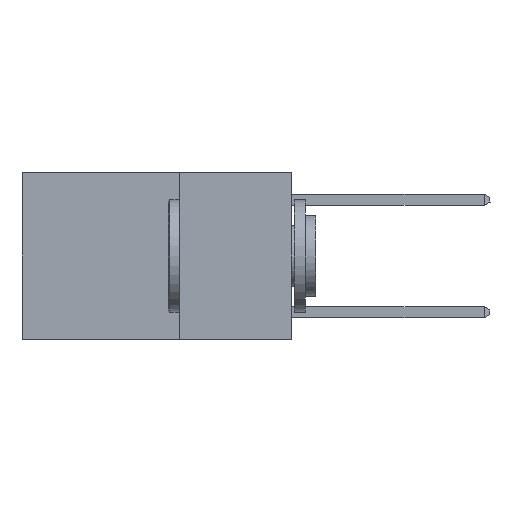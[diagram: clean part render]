
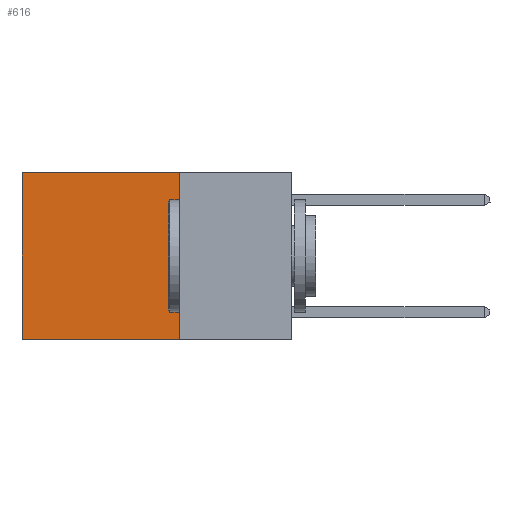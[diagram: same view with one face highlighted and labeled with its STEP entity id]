
A CAD part, left-side view. The second image highlights one B-rep face of the part: STEP entity #616.
In plain terms, the highlighted planar face has unit normal (-1, 0, 0).
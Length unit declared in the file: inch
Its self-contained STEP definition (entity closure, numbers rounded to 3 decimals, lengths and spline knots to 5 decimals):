
#616 = ADVANCED_FACE ( 'NONE', ( #10495 ), #8741, .F. ) ;
#1155 = DIRECTION ( 'NONE',  ( 1., 0., 0. ) ) ;
#2367 = DIRECTION ( 'NONE',  ( 0., 0., -1. ) ) ;
#2656 = LINE ( 'NONE', #16174, #15513 ) ;
#3738 = CARTESIAN_POINT ( 'NONE',  ( 0.2625, 0.6, 0. ) ) ;
#3993 = EDGE_CURVE ( 'NONE', #8483, #4294, #12483, .T. ) ;
#4294 = VERTEX_POINT ( 'NONE', #6613 ) ;
#4407 = AXIS2_PLACEMENT_3D ( 'NONE', #13640, #1155, #17614 ) ;
#5126 = CARTESIAN_POINT ( 'NONE',  ( 0.2625, 0.6, 0. ) ) ;
#6286 = ORIENTED_EDGE ( 'NONE', *, *, #8292, .T. ) ;
#6333 = DIRECTION ( 'NONE',  ( 0., 0., -1. ) ) ;
#6613 = CARTESIAN_POINT ( 'NONE',  ( 0.2625, 0.25, -0.37 ) ) ;
#6821 = EDGE_LOOP ( 'NONE', ( #9517, #14173, #14596, #6286 ) ) ;
#7365 = VECTOR ( 'NONE', #2367, 39.37008 ) ;
#7844 = VECTOR ( 'NONE', #6333, 39.37008 ) ;
#8292 = EDGE_CURVE ( 'NONE', #8483, #14912, #2656, .T. ) ;
#8483 = VERTEX_POINT ( 'NONE', #10400 ) ;
#8741 = PLANE ( 'NONE',  #4407 ) ;
#9517 = ORIENTED_EDGE ( 'NONE', *, *, #13443, .T. ) ;
#10400 = CARTESIAN_POINT ( 'NONE',  ( 0.2625, 0.25, 0. ) ) ;
#10495 = FACE_OUTER_BOUND ( 'NONE', #6821, .T. ) ;
#12483 = LINE ( 'NONE', #13733, #7844 ) ;
#13443 = EDGE_CURVE ( 'NONE', #14912, #16844, #15970, .T. ) ;
#13478 = DIRECTION ( 'NONE',  ( 0., 1., 0. ) ) ;
#13640 = CARTESIAN_POINT ( 'NONE',  ( 0.2625, 0.25, 0. ) ) ;
#13733 = CARTESIAN_POINT ( 'NONE',  ( 0.2625, 0.25, 0. ) ) ;
#13985 = VECTOR ( 'NONE', #14720, 39.37008 ) ;
#14173 = ORIENTED_EDGE ( 'NONE', *, *, #16474, .F. ) ;
#14596 = ORIENTED_EDGE ( 'NONE', *, *, #3993, .F. ) ;
#14720 = DIRECTION ( 'NONE',  ( 0., 1., 0. ) ) ;
#14793 = CARTESIAN_POINT ( 'NONE',  ( 0.2625, 0.6, -0.37 ) ) ;
#14912 = VERTEX_POINT ( 'NONE', #5126 ) ;
#15177 = LINE ( 'NONE', #18305, #13985 ) ;
#15513 = VECTOR ( 'NONE', #13478, 39.37008 ) ;
#15970 = LINE ( 'NONE', #3738, #7365 ) ;
#16174 = CARTESIAN_POINT ( 'NONE',  ( 0.2625, 0.25, 0. ) ) ;
#16474 = EDGE_CURVE ( 'NONE', #4294, #16844, #15177, .T. ) ;
#16844 = VERTEX_POINT ( 'NONE', #14793 ) ;
#17614 = DIRECTION ( 'NONE',  ( 0., 0., -1. ) ) ;
#18305 = CARTESIAN_POINT ( 'NONE',  ( 0.2625, 0.25, -0.37 ) ) ;
